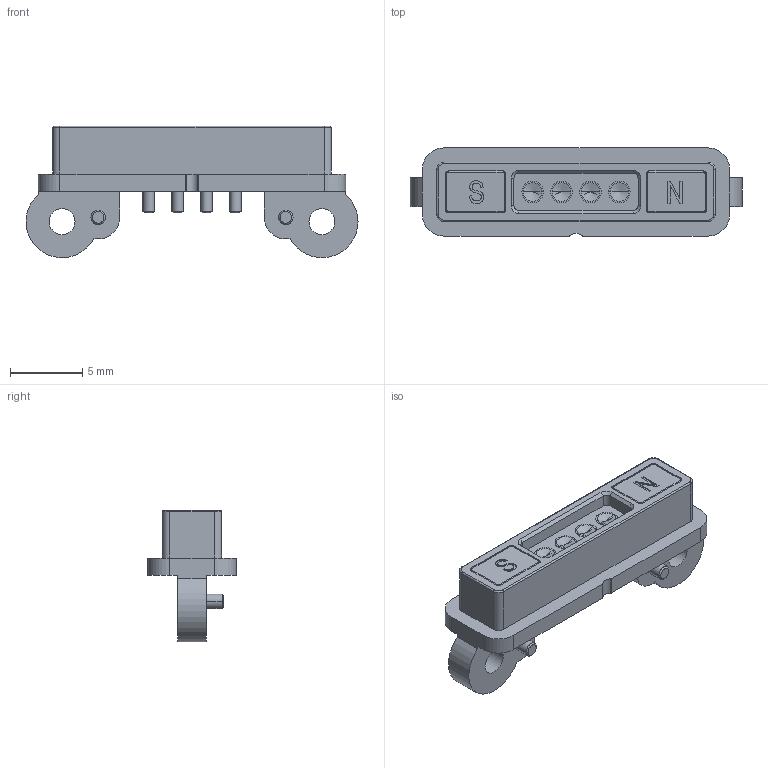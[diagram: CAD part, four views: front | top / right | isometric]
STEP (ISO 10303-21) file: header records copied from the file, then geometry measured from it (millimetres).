
FILE_DESCRIPTION (( 'STEP AP203' ), '1' );
FILE_NAME ('686-J0421251124.STEP', '2023-03-01T11:03:47', ( 'Magnum' ), ( '' ), 'SwSTEP 2.0', 'SolidWorks 2020', '' );
FILE_SCHEMA (( 'CONFIG_CONTROL_DESIGN' ));
Length unit declared in the file: millimetre
Products named in the file (1): 686-J0421251124
Bounding box: 23 x 6.1 x 9.09 mm (x, y, z)
Volume: 446.9 mm3; surface area: 762.4 mm2
Topology: 5 solids, 7 shells, 246 faces, 587 edges, 368 vertices
Faces by surface type: plane 94, cylinder 88, cone 30, bspline 28, torus 6
Entity records: 8052 total; most frequent: CARTESIAN_POINT 2286, DIRECTION 1203, ORIENTED_EDGE 1158, EDGE_CURVE 579, AXIS2_PLACEMENT_3D 445, VERTEX_POINT 368, LINE 313, VECTOR 313
